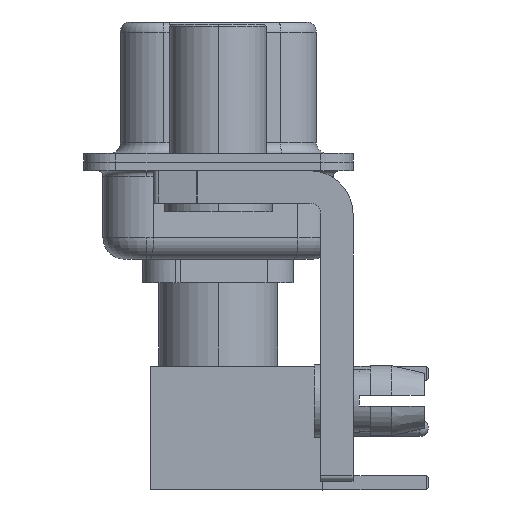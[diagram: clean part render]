
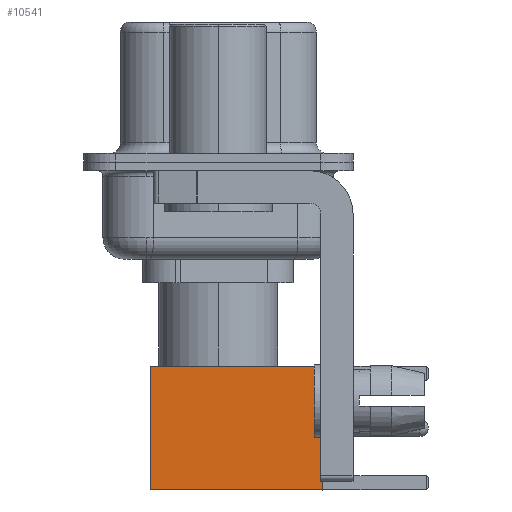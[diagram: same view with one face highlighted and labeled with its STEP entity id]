
A CAD part, left-side view. The second image highlights one B-rep face of the part: STEP entity #10541.
In plain terms, the highlighted face is planar.
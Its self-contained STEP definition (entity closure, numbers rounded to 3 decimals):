
#2230 = ORIENTED_EDGE ( 'NONE', *, *, #6632, .T. ) ;
#2792 = CARTESIAN_POINT ( 'NONE',  ( 2.875, 2.875, 0. ) ) ;
#2960 = ORIENTED_EDGE ( 'NONE', *, *, #6253, .F. ) ;
#3076 = VECTOR ( 'NONE', #22561, 1000. ) ;
#3086 = VERTEX_POINT ( 'NONE', #2792 ) ;
#3615 = CARTESIAN_POINT ( 'NONE',  ( -2.875, 2.875, 0. ) ) ;
#5079 = DIRECTION ( 'NONE',  ( 0., 0., 1. ) ) ;
#6136 = LINE ( 'NONE', #18291, #24094 ) ;
#6212 = CARTESIAN_POINT ( 'NONE',  ( 0., 2.875, 0. ) ) ;
#6253 = EDGE_CURVE ( 'NONE', #9386, #18331, #24649, .T. ) ;
#6285 = EDGE_CURVE ( 'NONE', #8018, #9386, #20859, .T. ) ;
#6627 = CARTESIAN_POINT ( 'NONE',  ( 0., 2.875, 8. ) ) ;
#6632 = EDGE_CURVE ( 'NONE', #3086, #18331, #17843, .T. ) ;
#6753 = DIRECTION ( 'NONE',  ( -1., 0., 0. ) ) ;
#6854 = ORIENTED_EDGE ( 'NONE', *, *, #23398, .T. ) ;
#7042 = FACE_OUTER_BOUND ( 'NONE', #20445, .T. ) ;
#8003 = ORIENTED_EDGE ( 'NONE', *, *, #6285, .F. ) ;
#8018 = VERTEX_POINT ( 'NONE', #10831 ) ;
#9224 = CARTESIAN_POINT ( 'NONE',  ( -2.875, 2.875, 0. ) ) ;
#9249 = CARTESIAN_POINT ( 'NONE',  ( 2.875, 2.875, 0. ) ) ;
#9386 = VERTEX_POINT ( 'NONE', #16321 ) ;
#10541 = ADVANCED_FACE ( 'NONE', ( #7042 ), #15260, .T. ) ;
#10831 = CARTESIAN_POINT ( 'NONE',  ( 2.875, 2.875, 8. ) ) ;
#12340 = DIRECTION ( 'NONE',  ( -1., 0., 0. ) ) ;
#14344 = VECTOR ( 'NONE', #6753, 1000. ) ;
#15260 = PLANE ( 'NONE',  #19092 ) ;
#16321 = CARTESIAN_POINT ( 'NONE',  ( -2.875, 2.875, 8. ) ) ;
#17843 = LINE ( 'NONE', #6212, #20592 ) ;
#18291 = CARTESIAN_POINT ( 'NONE',  ( 2.875, 2.875, 0. ) ) ;
#18331 = VERTEX_POINT ( 'NONE', #3615 ) ;
#19092 = AXIS2_PLACEMENT_3D ( 'NONE', #9249, #23218, #5079 ) ;
#19516 = DIRECTION ( 'NONE',  ( 0., 0., -1. ) ) ;
#20445 = EDGE_LOOP ( 'NONE', ( #6854, #2230, #2960, #8003 ) ) ;
#20592 = VECTOR ( 'NONE', #12340, 1000. ) ;
#20859 = LINE ( 'NONE', #6627, #14344 ) ;
#22561 = DIRECTION ( 'NONE',  ( 0., 0., -1. ) ) ;
#23218 = DIRECTION ( 'NONE',  ( 0., 1., 0. ) ) ;
#23398 = EDGE_CURVE ( 'NONE', #8018, #3086, #6136, .T. ) ;
#24094 = VECTOR ( 'NONE', #19516, 1000. ) ;
#24649 = LINE ( 'NONE', #9224, #3076 ) ;
